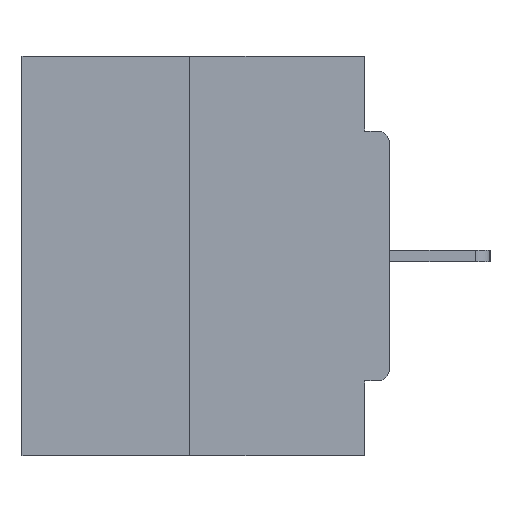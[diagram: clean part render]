
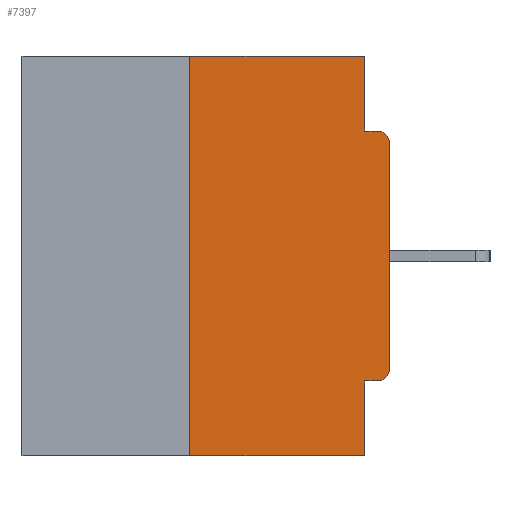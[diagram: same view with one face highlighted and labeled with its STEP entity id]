
A CAD part, left-side view. The second image highlights one B-rep face of the part: STEP entity #7397.
In plain terms, the highlighted planar face has unit normal (-1, 0, 0).
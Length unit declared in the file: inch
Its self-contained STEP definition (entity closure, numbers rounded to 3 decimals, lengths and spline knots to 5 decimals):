
#33 = VECTOR ( 'NONE', #34358, 39.37008 ) ;
#376 = EDGE_LOOP ( 'NONE', ( #17765, #21695, #31877, #40014, #16340, #1590, #18282, #4550, #6510, #23145 ) ) ;
#693 = DIRECTION ( 'NONE',  ( 0., 0., 1. ) ) ;
#697 = LINE ( 'NONE', #8850, #16451 ) ;
#840 = VECTOR ( 'NONE', #10288, 39.37008 ) ;
#1590 = ORIENTED_EDGE ( 'NONE', *, *, #9768, .T. ) ;
#1836 = LINE ( 'NONE', #32073, #840 ) ;
#2720 = VERTEX_POINT ( 'NONE', #12148 ) ;
#2779 = EDGE_CURVE ( 'NONE', #25088, #25079, #30833, .T. ) ;
#3362 = DIRECTION ( 'NONE',  ( 0., -1., 0. ) ) ;
#3507 = EDGE_CURVE ( 'NONE', #25088, #31448, #4419, .T. ) ;
#3533 = CARTESIAN_POINT ( 'NONE',  ( 0., 0.25, -0.5 ) ) ;
#3881 = VERTEX_POINT ( 'NONE', #30857 ) ;
#4419 = LINE ( 'NONE', #36560, #11843 ) ;
#4550 = ORIENTED_EDGE ( 'NONE', *, *, #40228, .T. ) ;
#4577 = DIRECTION ( 'NONE',  ( 0., 0., -1. ) ) ;
#4757 = CARTESIAN_POINT ( 'NONE',  ( 0., 0.031, -0.4065 ) ) ;
#5250 = VERTEX_POINT ( 'NONE', #30721 ) ;
#5977 = DIRECTION ( 'NONE',  ( 0., 0., -1. ) ) ;
#6112 = DIRECTION ( 'NONE',  ( 1., 0., 0. ) ) ;
#6155 = PLANE ( 'NONE',  #29155 ) ;
#6279 = CARTESIAN_POINT ( 'NONE',  ( 0., 0.031, -0.5 ) ) ;
#6510 = ORIENTED_EDGE ( 'NONE', *, *, #39973, .F. ) ;
#7397 = ADVANCED_FACE ( 'NONE', ( #10534 ), #6155, .F. ) ;
#7806 = VERTEX_POINT ( 'NONE', #32846 ) ;
#8050 = CARTESIAN_POINT ( 'NONE',  ( 0., 0.46, 0. ) ) ;
#8850 = CARTESIAN_POINT ( 'NONE',  ( 0., 0., -0.4065 ) ) ;
#9335 = VECTOR ( 'NONE', #4577, 39.37008 ) ;
#9768 = EDGE_CURVE ( 'NONE', #38711, #3881, #36140, .T. ) ;
#9918 = CARTESIAN_POINT ( 'NONE',  ( 0., 0.015, -0.3915 ) ) ;
#9946 = CIRCLE ( 'NONE', #31828, 0.015 ) ;
#10288 = DIRECTION ( 'NONE',  ( 0., -1., 0. ) ) ;
#10399 = LINE ( 'NONE', #6279, #33 ) ;
#10534 = FACE_OUTER_BOUND ( 'NONE', #376, .T. ) ;
#11099 = CARTESIAN_POINT ( 'NONE',  ( 0., 0.015, -0.1085 ) ) ;
#11482 = VECTOR ( 'NONE', #3362, 39.37008 ) ;
#11843 = VECTOR ( 'NONE', #32980, 39.37008 ) ;
#12148 = CARTESIAN_POINT ( 'NONE',  ( 0., 0.031, 0. ) ) ;
#13066 = DIRECTION ( 'NONE',  ( 0., 0., -1. ) ) ;
#13603 = VECTOR ( 'NONE', #693, 39.37008 ) ;
#14242 = DIRECTION ( 'NONE',  ( 0., 0., -1. ) ) ;
#16340 = ORIENTED_EDGE ( 'NONE', *, *, #17676, .F. ) ;
#16451 = VECTOR ( 'NONE', #30598, 39.37008 ) ;
#17634 = LINE ( 'NONE', #23308, #9335 ) ;
#17676 = EDGE_CURVE ( 'NONE', #38711, #19969, #697, .T. ) ;
#17765 = ORIENTED_EDGE ( 'NONE', *, *, #36600, .F. ) ;
#18282 = ORIENTED_EDGE ( 'NONE', *, *, #30952, .T. ) ;
#19638 = CARTESIAN_POINT ( 'NONE',  ( 0., 0., 0. ) ) ;
#19673 = EDGE_CURVE ( 'NONE', #19969, #25079, #10399, .T. ) ;
#19755 = LINE ( 'NONE', #37522, #11482 ) ;
#19969 = VERTEX_POINT ( 'NONE', #4757 ) ;
#21695 = ORIENTED_EDGE ( 'NONE', *, *, #3507, .F. ) ;
#23145 = ORIENTED_EDGE ( 'NONE', *, *, #35562, .F. ) ;
#23308 = CARTESIAN_POINT ( 'NONE',  ( 0., 0.031, 0. ) ) ;
#25079 = VERTEX_POINT ( 'NONE', #28378 ) ;
#25088 = VERTEX_POINT ( 'NONE', #3533 ) ;
#25166 = CARTESIAN_POINT ( 'NONE',  ( 0., 0.25, 0. ) ) ;
#26242 = CARTESIAN_POINT ( 'NONE',  ( 0., 0.031, -0.0935 ) ) ;
#27157 = AXIS2_PLACEMENT_3D ( 'NONE', #9918, #31684, #13066 ) ;
#27685 = VERTEX_POINT ( 'NONE', #26242 ) ;
#28378 = CARTESIAN_POINT ( 'NONE',  ( 0., 0.031, -0.5 ) ) ;
#29155 = AXIS2_PLACEMENT_3D ( 'NONE', #8050, #6112, #5977 ) ;
#29855 = VECTOR ( 'NONE', #30065, 39.37008 ) ;
#30065 = DIRECTION ( 'NONE',  ( 0., -1., 0. ) ) ;
#30598 = DIRECTION ( 'NONE',  ( 0., 1., 0. ) ) ;
#30721 = CARTESIAN_POINT ( 'NONE',  ( 0., 0.015, -0.0935 ) ) ;
#30833 = LINE ( 'NONE', #31007, #29855 ) ;
#30857 = CARTESIAN_POINT ( 'NONE',  ( 0., 0., -0.3915 ) ) ;
#30952 = EDGE_CURVE ( 'NONE', #3881, #7806, #38313, .T. ) ;
#31007 = CARTESIAN_POINT ( 'NONE',  ( 0., 0.46, -0.5 ) ) ;
#31448 = VERTEX_POINT ( 'NONE', #25166 ) ;
#31684 = DIRECTION ( 'NONE',  ( -1., 0., 0. ) ) ;
#31828 = AXIS2_PLACEMENT_3D ( 'NONE', #11099, #32861, #14242 ) ;
#31877 = ORIENTED_EDGE ( 'NONE', *, *, #2779, .T. ) ;
#32073 = CARTESIAN_POINT ( 'NONE',  ( 0., 0.46, 0. ) ) ;
#32846 = CARTESIAN_POINT ( 'NONE',  ( 0., 0., -0.1085 ) ) ;
#32861 = DIRECTION ( 'NONE',  ( -1., 0., 0. ) ) ;
#32980 = DIRECTION ( 'NONE',  ( 0., 0., 1. ) ) ;
#34358 = DIRECTION ( 'NONE',  ( 0., 0., -1. ) ) ;
#35562 = EDGE_CURVE ( 'NONE', #2720, #27685, #17634, .T. ) ;
#36140 = CIRCLE ( 'NONE', #27157, 0.015 ) ;
#36560 = CARTESIAN_POINT ( 'NONE',  ( 0., 0.25, 0. ) ) ;
#36600 = EDGE_CURVE ( 'NONE', #31448, #2720, #1836, .T. ) ;
#36826 = CARTESIAN_POINT ( 'NONE',  ( 0., 0.015, -0.4065 ) ) ;
#37522 = CARTESIAN_POINT ( 'NONE',  ( 0., 0., -0.0935 ) ) ;
#38313 = LINE ( 'NONE', #19638, #13603 ) ;
#38711 = VERTEX_POINT ( 'NONE', #36826 ) ;
#39973 = EDGE_CURVE ( 'NONE', #27685, #5250, #19755, .T. ) ;
#40014 = ORIENTED_EDGE ( 'NONE', *, *, #19673, .F. ) ;
#40228 = EDGE_CURVE ( 'NONE', #7806, #5250, #9946, .T. ) ;
